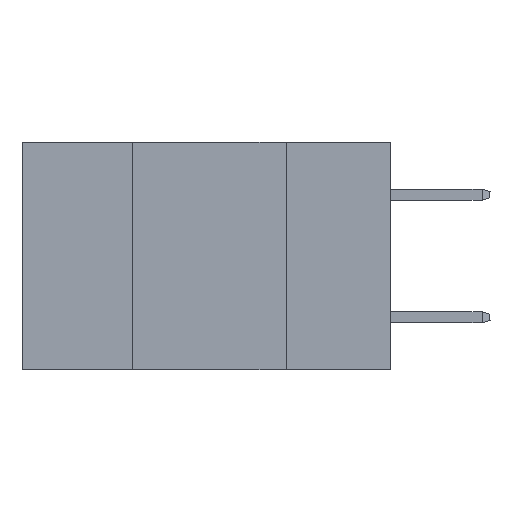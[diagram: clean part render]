
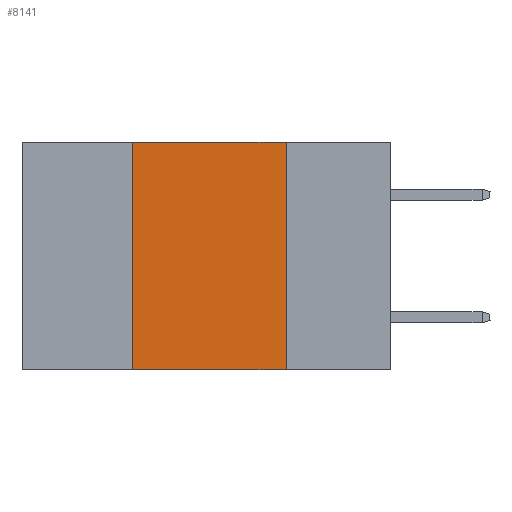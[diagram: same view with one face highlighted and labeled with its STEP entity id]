
A CAD part, left-side view. The second image highlights one B-rep face of the part: STEP entity #8141.
In plain terms, the highlighted planar face has unit normal (-1, 0, 0).
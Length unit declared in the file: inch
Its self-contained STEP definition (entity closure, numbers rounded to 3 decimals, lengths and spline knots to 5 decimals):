
#39 = AXIS2_PLACEMENT_3D ( 'NONE', #1739, #1704, #10929 ) ;
#298 = LINE ( 'NONE', #1257, #9693 ) ;
#601 = VECTOR ( 'NONE', #10252, 39.37008 ) ;
#1257 = CARTESIAN_POINT ( 'NONE',  ( 0., 0.17, 0. ) ) ;
#1704 = DIRECTION ( 'NONE',  ( 1., 0., 0. ) ) ;
#1739 = CARTESIAN_POINT ( 'NONE',  ( 0., 0.6, 0. ) ) ;
#1776 = CARTESIAN_POINT ( 'NONE',  ( 0., 0.42, 0. ) ) ;
#2057 = FACE_OUTER_BOUND ( 'NONE', #2211, .T. ) ;
#2211 = EDGE_LOOP ( 'NONE', ( #4462, #6149, #5220, #8801 ) ) ;
#3141 = VECTOR ( 'NONE', #7545, 39.37008 ) ;
#3142 = DIRECTION ( 'NONE',  ( 0., 0., -1. ) ) ;
#3835 = EDGE_CURVE ( 'NONE', #9843, #8031, #298, .T. ) ;
#4116 = LINE ( 'NONE', #7788, #5703 ) ;
#4415 = VERTEX_POINT ( 'NONE', #6902 ) ;
#4440 = CARTESIAN_POINT ( 'NONE',  ( 0., 0.42, 0. ) ) ;
#4462 = ORIENTED_EDGE ( 'NONE', *, *, #3835, .F. ) ;
#5220 = ORIENTED_EDGE ( 'NONE', *, *, #8375, .F. ) ;
#5703 = VECTOR ( 'NONE', #10302, 39.37008 ) ;
#6149 = ORIENTED_EDGE ( 'NONE', *, *, #6967, .F. ) ;
#6532 = CARTESIAN_POINT ( 'NONE',  ( 0., 0.17, 0. ) ) ;
#6711 = LINE ( 'NONE', #1776, #601 ) ;
#6902 = CARTESIAN_POINT ( 'NONE',  ( 0., 0.42, -0.37 ) ) ;
#6967 = EDGE_CURVE ( 'NONE', #8380, #9843, #4116, .T. ) ;
#7545 = DIRECTION ( 'NONE',  ( 0., -1., 0. ) ) ;
#7788 = CARTESIAN_POINT ( 'NONE',  ( 0., 0.6, 0. ) ) ;
#8031 = VERTEX_POINT ( 'NONE', #10896 ) ;
#8141 = ADVANCED_FACE ( 'NONE', ( #2057 ), #10134, .F. ) ;
#8375 = EDGE_CURVE ( 'NONE', #4415, #8380, #6711, .T. ) ;
#8380 = VERTEX_POINT ( 'NONE', #4440 ) ;
#8658 = EDGE_CURVE ( 'NONE', #4415, #8031, #9464, .T. ) ;
#8801 = ORIENTED_EDGE ( 'NONE', *, *, #8658, .T. ) ;
#9464 = LINE ( 'NONE', #10025, #3141 ) ;
#9693 = VECTOR ( 'NONE', #3142, 39.37008 ) ;
#9843 = VERTEX_POINT ( 'NONE', #6532 ) ;
#10025 = CARTESIAN_POINT ( 'NONE',  ( 0., 0.6, -0.37 ) ) ;
#10134 = PLANE ( 'NONE',  #39 ) ;
#10252 = DIRECTION ( 'NONE',  ( 0., 0., 1. ) ) ;
#10302 = DIRECTION ( 'NONE',  ( 0., -1., 0. ) ) ;
#10896 = CARTESIAN_POINT ( 'NONE',  ( 0., 0.17, -0.37 ) ) ;
#10929 = DIRECTION ( 'NONE',  ( 0., 0., -1. ) ) ;
